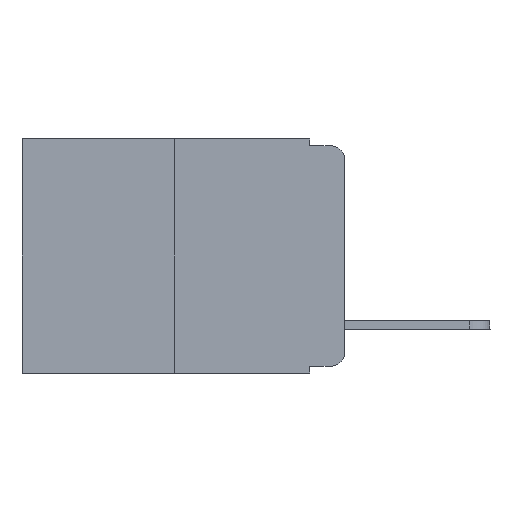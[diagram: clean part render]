
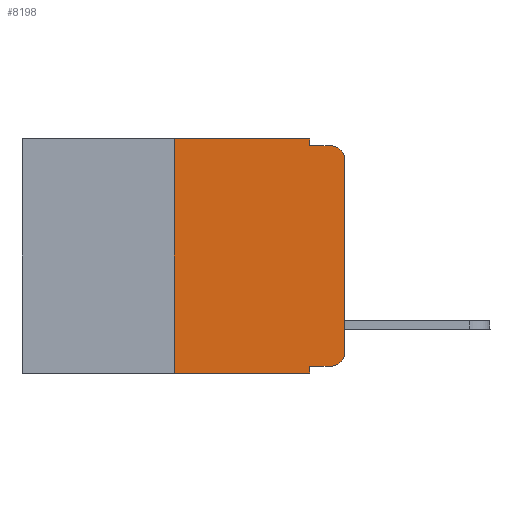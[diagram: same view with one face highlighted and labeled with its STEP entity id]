
A CAD part, left-side view. The second image highlights one B-rep face of the part: STEP entity #8198.
In plain terms, the highlighted planar face has unit normal (-1, 0, 0).
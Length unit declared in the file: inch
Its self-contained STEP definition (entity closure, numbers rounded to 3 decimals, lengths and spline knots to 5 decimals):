
#233 = ORIENTED_EDGE ( 'NONE', *, *, #10672, .F. ) ;
#245 = DIRECTION ( 'NONE',  ( 0., -1., 0. ) ) ;
#260 = DIRECTION ( 'NONE',  ( 0., 0., -1. ) ) ;
#275 = CARTESIAN_POINT ( 'NONE',  ( 0., 0.051, -0.01 ) ) ;
#398 = DIRECTION ( 'NONE',  ( 0., 0., 1. ) ) ;
#546 = DIRECTION ( 'NONE',  ( -1., 0., 0. ) ) ;
#1035 = VECTOR ( 'NONE', #3988, 39.37008 ) ;
#1243 = CIRCLE ( 'NONE', #5018, 0.02 ) ;
#1361 = DIRECTION ( 'NONE',  ( 0., 0., -1. ) ) ;
#1499 = CARTESIAN_POINT ( 'NONE',  ( 0., 0.02, -0.03 ) ) ;
#1741 = CARTESIAN_POINT ( 'NONE',  ( 0., 0.051, -0.333 ) ) ;
#1766 = DIRECTION ( 'NONE',  ( 0., -1., 0. ) ) ;
#2267 = CARTESIAN_POINT ( 'NONE',  ( 0., 0., 0. ) ) ;
#2640 = LINE ( 'NONE', #1741, #12263 ) ;
#3053 = EDGE_CURVE ( 'NONE', #3065, #12557, #1243, .T. ) ;
#3065 = VERTEX_POINT ( 'NONE', #13431 ) ;
#3080 = DIRECTION ( 'NONE',  ( 1., 0., 0. ) ) ;
#3245 = VECTOR ( 'NONE', #1766, 39.37008 ) ;
#3263 = VECTOR ( 'NONE', #245, 39.37008 ) ;
#3364 = ORIENTED_EDGE ( 'NONE', *, *, #3053, .T. ) ;
#3396 = CARTESIAN_POINT ( 'NONE',  ( 0., 0.051, 0. ) ) ;
#3445 = EDGE_CURVE ( 'NONE', #8230, #9101, #6132, .T. ) ;
#3481 = EDGE_CURVE ( 'NONE', #5739, #6797, #4887, .T. ) ;
#3530 = VECTOR ( 'NONE', #398, 39.37008 ) ;
#3595 = LINE ( 'NONE', #3396, #12149 ) ;
#3781 = CARTESIAN_POINT ( 'NONE',  ( 0., 0.051, 0. ) ) ;
#3811 = CARTESIAN_POINT ( 'NONE',  ( 0., 0.02, -0.313 ) ) ;
#3921 = CARTESIAN_POINT ( 'NONE',  ( 0., 0.051, -0.01 ) ) ;
#3988 = DIRECTION ( 'NONE',  ( 0., -1., 0. ) ) ;
#4013 = ORIENTED_EDGE ( 'NONE', *, *, #7007, .F. ) ;
#4201 = ORIENTED_EDGE ( 'NONE', *, *, #12167, .T. ) ;
#4375 = VECTOR ( 'NONE', #9383, 39.37008 ) ;
#4587 = CIRCLE ( 'NONE', #5467, 0.02 ) ;
#4887 = LINE ( 'NONE', #7047, #3245 ) ;
#5018 = AXIS2_PLACEMENT_3D ( 'NONE', #3811, #546, #10987 ) ;
#5112 = ORIENTED_EDGE ( 'NONE', *, *, #3481, .F. ) ;
#5185 = CARTESIAN_POINT ( 'NONE',  ( 0., 0., -0.03 ) ) ;
#5467 = AXIS2_PLACEMENT_3D ( 'NONE', #1499, #9926, #9857 ) ;
#5739 = VERTEX_POINT ( 'NONE', #6783 ) ;
#5749 = CARTESIAN_POINT ( 'NONE',  ( 0., 0.051, -0.333 ) ) ;
#6056 = VERTEX_POINT ( 'NONE', #5185 ) ;
#6132 = LINE ( 'NONE', #3921, #1035 ) ;
#6552 = EDGE_LOOP ( 'NONE', ( #4201, #10656, #7781, #13412, #5112, #4013, #11464, #233, #12643, #3364 ) ) ;
#6783 = CARTESIAN_POINT ( 'NONE',  ( 0., 0.25, 0. ) ) ;
#6797 = VERTEX_POINT ( 'NONE', #9408 ) ;
#6942 = DIRECTION ( 'NONE',  ( 0., -1., 0. ) ) ;
#7007 = EDGE_CURVE ( 'NONE', #11635, #5739, #10642, .T. ) ;
#7047 = CARTESIAN_POINT ( 'NONE',  ( 0., 0.473, 0. ) ) ;
#7306 = LINE ( 'NONE', #2267, #4375 ) ;
#7336 = DIRECTION ( 'NONE',  ( 0., 0., -1. ) ) ;
#7454 = VECTOR ( 'NONE', #1361, 39.37008 ) ;
#7573 = LINE ( 'NONE', #8879, #3263 ) ;
#7781 = ORIENTED_EDGE ( 'NONE', *, *, #3445, .F. ) ;
#8198 = ADVANCED_FACE ( 'NONE', ( #9411 ), #13661, .F. ) ;
#8230 = VERTEX_POINT ( 'NONE', #275 ) ;
#8380 = CARTESIAN_POINT ( 'NONE',  ( 0., 0.473, 0. ) ) ;
#8626 = CARTESIAN_POINT ( 'NONE',  ( 0., 0.25, 0. ) ) ;
#8879 = CARTESIAN_POINT ( 'NONE',  ( 0., 0.473, -0.343 ) ) ;
#9019 = EDGE_CURVE ( 'NONE', #11956, #3065, #2640, .T. ) ;
#9101 = VERTEX_POINT ( 'NONE', #9326 ) ;
#9326 = CARTESIAN_POINT ( 'NONE',  ( 0., 0.02, -0.01 ) ) ;
#9383 = DIRECTION ( 'NONE',  ( 0., 0., 1. ) ) ;
#9408 = CARTESIAN_POINT ( 'NONE',  ( 0., 0.051, 0. ) ) ;
#9411 = FACE_OUTER_BOUND ( 'NONE', #6552, .T. ) ;
#9857 = DIRECTION ( 'NONE',  ( 0., 0., -1. ) ) ;
#9926 = DIRECTION ( 'NONE',  ( -1., 0., 0. ) ) ;
#10642 = LINE ( 'NONE', #8626, #3530 ) ;
#10656 = ORIENTED_EDGE ( 'NONE', *, *, #11125, .T. ) ;
#10672 = EDGE_CURVE ( 'NONE', #11956, #11542, #3595, .T. ) ;
#10777 = CARTESIAN_POINT ( 'NONE',  ( 0., 0., -0.313 ) ) ;
#10889 = LINE ( 'NONE', #3781, #7454 ) ;
#10987 = DIRECTION ( 'NONE',  ( 0., 0., -1. ) ) ;
#11103 = EDGE_CURVE ( 'NONE', #11635, #11542, #7573, .T. ) ;
#11125 = EDGE_CURVE ( 'NONE', #6056, #9101, #4587, .T. ) ;
#11422 = CARTESIAN_POINT ( 'NONE',  ( 0., 0.25, -0.343 ) ) ;
#11464 = ORIENTED_EDGE ( 'NONE', *, *, #11103, .T. ) ;
#11542 = VERTEX_POINT ( 'NONE', #13100 ) ;
#11635 = VERTEX_POINT ( 'NONE', #11422 ) ;
#11956 = VERTEX_POINT ( 'NONE', #5749 ) ;
#12149 = VECTOR ( 'NONE', #260, 39.37008 ) ;
#12167 = EDGE_CURVE ( 'NONE', #12557, #6056, #7306, .T. ) ;
#12263 = VECTOR ( 'NONE', #6942, 39.37008 ) ;
#12557 = VERTEX_POINT ( 'NONE', #10777 ) ;
#12643 = ORIENTED_EDGE ( 'NONE', *, *, #9019, .T. ) ;
#13100 = CARTESIAN_POINT ( 'NONE',  ( 0., 0.051, -0.343 ) ) ;
#13144 = AXIS2_PLACEMENT_3D ( 'NONE', #8380, #3080, #7336 ) ;
#13412 = ORIENTED_EDGE ( 'NONE', *, *, #13588, .F. ) ;
#13431 = CARTESIAN_POINT ( 'NONE',  ( 0., 0.02, -0.333 ) ) ;
#13588 = EDGE_CURVE ( 'NONE', #6797, #8230, #10889, .T. ) ;
#13661 = PLANE ( 'NONE',  #13144 ) ;
